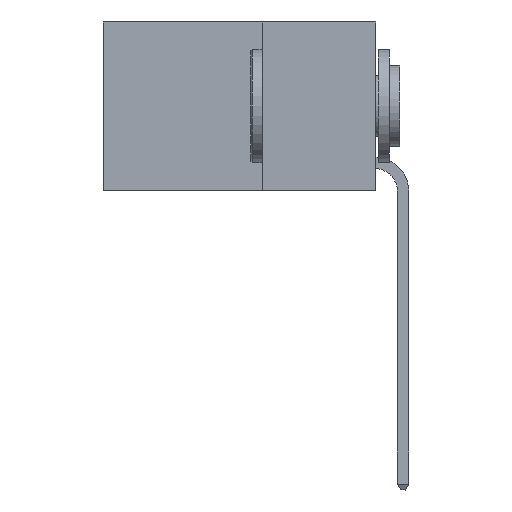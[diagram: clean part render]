
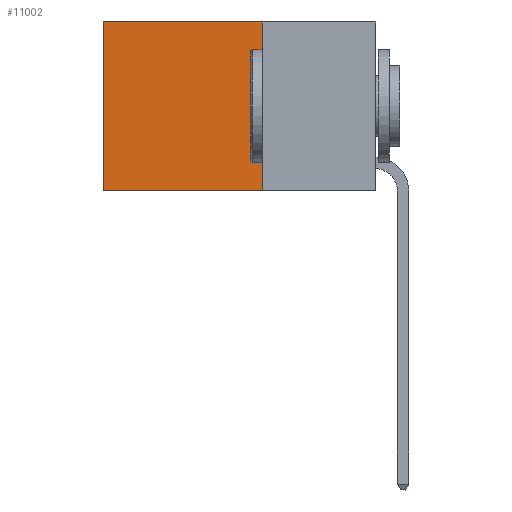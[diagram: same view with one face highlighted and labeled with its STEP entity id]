
A CAD part, left-side view. The second image highlights one B-rep face of the part: STEP entity #11002.
In plain terms, the highlighted planar face has unit normal (-1, 0, 0).
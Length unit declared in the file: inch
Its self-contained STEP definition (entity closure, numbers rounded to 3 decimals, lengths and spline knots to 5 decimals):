
#1043 = CARTESIAN_POINT ( 'NONE',  ( 0.2625, 0.25, -0.37 ) ) ;
#1509 = DIRECTION ( 'NONE',  ( 0., 1., 0. ) ) ;
#1622 = CARTESIAN_POINT ( 'NONE',  ( 0.2625, 0.6, 0. ) ) ;
#1693 = ORIENTED_EDGE ( 'NONE', *, *, #9507, .F. ) ;
#1724 = CARTESIAN_POINT ( 'NONE',  ( 0.2625, 0.6, 0. ) ) ;
#2351 = CARTESIAN_POINT ( 'NONE',  ( 0.2625, 0.25, 0. ) ) ;
#2360 = AXIS2_PLACEMENT_3D ( 'NONE', #2351, #15853, #8600 ) ;
#3198 = DIRECTION ( 'NONE',  ( 0., 1., 0. ) ) ;
#3316 = VECTOR ( 'NONE', #1509, 39.37008 ) ;
#4209 = VECTOR ( 'NONE', #3198, 39.37008 ) ;
#4963 = ORIENTED_EDGE ( 'NONE', *, *, #11489, .F. ) ;
#5359 = VECTOR ( 'NONE', #12848, 39.37008 ) ;
#6451 = CARTESIAN_POINT ( 'NONE',  ( 0.2625, 0.25, 0. ) ) ;
#6600 = VECTOR ( 'NONE', #13779, 39.37008 ) ;
#6981 = LINE ( 'NONE', #6451, #6600 ) ;
#7063 = EDGE_LOOP ( 'NONE', ( #13350, #4963, #1693, #11310 ) ) ;
#7489 = VERTEX_POINT ( 'NONE', #10406 ) ;
#8600 = DIRECTION ( 'NONE',  ( 0., 0., -1. ) ) ;
#8646 = LINE ( 'NONE', #1622, #5359 ) ;
#8972 = CARTESIAN_POINT ( 'NONE',  ( 0.2625, 0.25, 0. ) ) ;
#9281 = CARTESIAN_POINT ( 'NONE',  ( 0.2625, 0.6, -0.37 ) ) ;
#9507 = EDGE_CURVE ( 'NONE', #7489, #10550, #6981, .T. ) ;
#9510 = EDGE_CURVE ( 'NONE', #7489, #10192, #12764, .T. ) ;
#10192 = VERTEX_POINT ( 'NONE', #1724 ) ;
#10272 = VERTEX_POINT ( 'NONE', #9281 ) ;
#10406 = CARTESIAN_POINT ( 'NONE',  ( 0.2625, 0.25, 0. ) ) ;
#10550 = VERTEX_POINT ( 'NONE', #1043 ) ;
#10577 = CARTESIAN_POINT ( 'NONE',  ( 0.2625, 0.25, -0.37 ) ) ;
#11002 = ADVANCED_FACE ( 'NONE', ( #13630 ), #14669, .F. ) ;
#11310 = ORIENTED_EDGE ( 'NONE', *, *, #9510, .T. ) ;
#11363 = EDGE_CURVE ( 'NONE', #10192, #10272, #8646, .T. ) ;
#11489 = EDGE_CURVE ( 'NONE', #10550, #10272, #13995, .T. ) ;
#12764 = LINE ( 'NONE', #8972, #3316 ) ;
#12848 = DIRECTION ( 'NONE',  ( 0., 0., -1. ) ) ;
#13350 = ORIENTED_EDGE ( 'NONE', *, *, #11363, .T. ) ;
#13630 = FACE_OUTER_BOUND ( 'NONE', #7063, .T. ) ;
#13779 = DIRECTION ( 'NONE',  ( 0., 0., -1. ) ) ;
#13995 = LINE ( 'NONE', #10577, #4209 ) ;
#14669 = PLANE ( 'NONE',  #2360 ) ;
#15853 = DIRECTION ( 'NONE',  ( 1., 0., 0. ) ) ;
